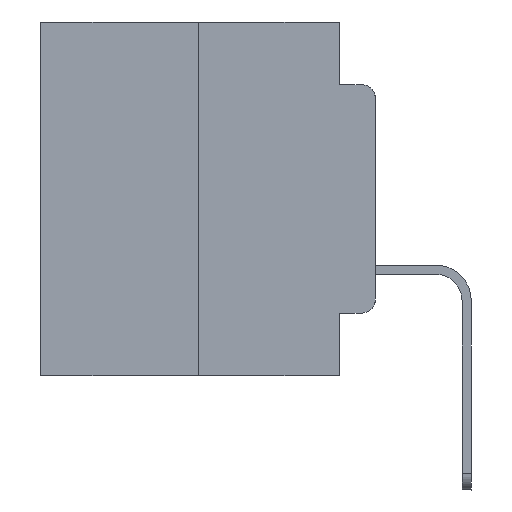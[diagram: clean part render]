
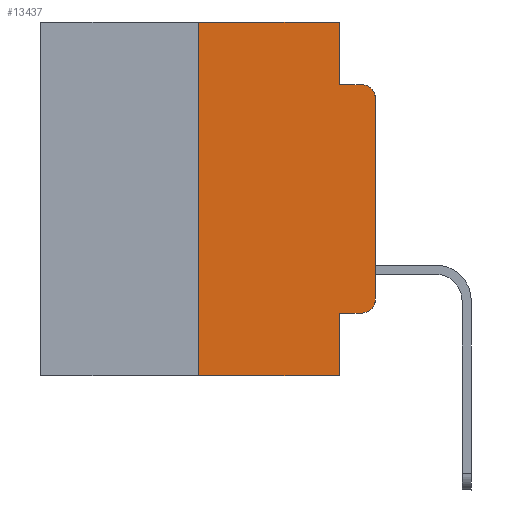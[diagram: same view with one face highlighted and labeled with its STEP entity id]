
A CAD part, left-side view. The second image highlights one B-rep face of the part: STEP entity #13437.
In plain terms, the highlighted planar face has unit normal (-1, 0, 0).
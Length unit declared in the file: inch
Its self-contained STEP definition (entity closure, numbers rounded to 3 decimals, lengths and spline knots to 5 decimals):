
#523 = CARTESIAN_POINT ( 'NONE',  ( 0., 0.02, -0.0885 ) ) ;
#645 = VECTOR ( 'NONE', #2696, 39.37008 ) ;
#682 = VERTEX_POINT ( 'NONE', #3819 ) ;
#1210 = VERTEX_POINT ( 'NONE', #19512 ) ;
#1734 = PLANE ( 'NONE',  #8685 ) ;
#1795 = EDGE_LOOP ( 'NONE', ( #7085, #4631, #19929, #17589, #19676, #7220, #11823, #26872, #26747, #7001 ) ) ;
#2447 = EDGE_CURVE ( 'NONE', #17027, #6965, #3572, .T. ) ;
#2696 = DIRECTION ( 'NONE',  ( 0., -1., 0. ) ) ;
#2859 = VERTEX_POINT ( 'NONE', #14136 ) ;
#2995 = VERTEX_POINT ( 'NONE', #21098 ) ;
#3008 = LINE ( 'NONE', #17358, #15386 ) ;
#3299 = EDGE_CURVE ( 'NONE', #2995, #1210, #4804, .T. ) ;
#3401 = DIRECTION ( 'NONE',  ( 0., -1., 0. ) ) ;
#3572 = LINE ( 'NONE', #23166, #25072 ) ;
#3819 = CARTESIAN_POINT ( 'NONE',  ( 0., 0.25, -0.5 ) ) ;
#4591 = CARTESIAN_POINT ( 'NONE',  ( 0., 0.02, -0.3915 ) ) ;
#4631 = ORIENTED_EDGE ( 'NONE', *, *, #19689, .T. ) ;
#4804 = LINE ( 'NONE', #20510, #16554 ) ;
#5043 = CARTESIAN_POINT ( 'NONE',  ( 0., 0.051, -0.0885 ) ) ;
#6478 = CIRCLE ( 'NONE', #6542, 0.02 ) ;
#6542 = AXIS2_PLACEMENT_3D ( 'NONE', #13864, #15934, #7295 ) ;
#6589 = EDGE_CURVE ( 'NONE', #17250, #19803, #21943, .T. ) ;
#6624 = EDGE_CURVE ( 'NONE', #2859, #8925, #10543, .T. ) ;
#6965 = VERTEX_POINT ( 'NONE', #19039 ) ;
#7001 = ORIENTED_EDGE ( 'NONE', *, *, #10308, .T. ) ;
#7067 = DIRECTION ( 'NONE',  ( 0., 0., -1. ) ) ;
#7085 = ORIENTED_EDGE ( 'NONE', *, *, #3299, .T. ) ;
#7220 = ORIENTED_EDGE ( 'NONE', *, *, #10747, .F. ) ;
#7295 = DIRECTION ( 'NONE',  ( 0., 0., -1. ) ) ;
#8685 = AXIS2_PLACEMENT_3D ( 'NONE', #9784, #13973, #9871 ) ;
#8925 = VERTEX_POINT ( 'NONE', #15623 ) ;
#9784 = CARTESIAN_POINT ( 'NONE',  ( 0., 0.473, 0. ) ) ;
#9871 = DIRECTION ( 'NONE',  ( 0., 0., -1. ) ) ;
#10241 = DIRECTION ( 'NONE',  ( 0., 0., 1. ) ) ;
#10308 = EDGE_CURVE ( 'NONE', #23856, #2995, #23254, .T. ) ;
#10543 = LINE ( 'NONE', #24446, #20632 ) ;
#10747 = EDGE_CURVE ( 'NONE', #682, #17027, #17678, .T. ) ;
#11102 = CARTESIAN_POINT ( 'NONE',  ( 0., 0.051, -0.4115 ) ) ;
#11119 = DIRECTION ( 'NONE',  ( 0., -1., 0. ) ) ;
#11823 = ORIENTED_EDGE ( 'NONE', *, *, #25903, .T. ) ;
#12394 = LINE ( 'NONE', #11102, #645 ) ;
#12458 = EDGE_CURVE ( 'NONE', #2859, #23856, #12394, .T. ) ;
#13437 = ADVANCED_FACE ( 'NONE', ( #26699 ), #1734, .F. ) ;
#13864 = CARTESIAN_POINT ( 'NONE',  ( 0., 0.02, -0.1085 ) ) ;
#13973 = DIRECTION ( 'NONE',  ( 1., 0., 0. ) ) ;
#14027 = DIRECTION ( 'NONE',  ( 0., 0., 1. ) ) ;
#14078 = DIRECTION ( 'NONE',  ( 0., 0., -1. ) ) ;
#14136 = CARTESIAN_POINT ( 'NONE',  ( 0., 0.051, -0.4115 ) ) ;
#14572 = LINE ( 'NONE', #15893, #24664 ) ;
#14951 = DIRECTION ( 'NONE',  ( 0., -1., 0. ) ) ;
#15386 = VECTOR ( 'NONE', #11119, 39.37008 ) ;
#15623 = CARTESIAN_POINT ( 'NONE',  ( 0., 0.051, -0.5 ) ) ;
#15893 = CARTESIAN_POINT ( 'NONE',  ( 0., 0.051, 0. ) ) ;
#15934 = DIRECTION ( 'NONE',  ( -1., 0., 0. ) ) ;
#16407 = VECTOR ( 'NONE', #3401, 39.37008 ) ;
#16450 = AXIS2_PLACEMENT_3D ( 'NONE', #4591, #19170, #7067 ) ;
#16554 = VECTOR ( 'NONE', #10241, 39.37008 ) ;
#16778 = CARTESIAN_POINT ( 'NONE',  ( 0., 0.25, 0. ) ) ;
#17027 = VERTEX_POINT ( 'NONE', #16778 ) ;
#17250 = VERTEX_POINT ( 'NONE', #22443 ) ;
#17358 = CARTESIAN_POINT ( 'NONE',  ( 0., 0.473, -0.5 ) ) ;
#17589 = ORIENTED_EDGE ( 'NONE', *, *, #20681, .F. ) ;
#17678 = LINE ( 'NONE', #25525, #22578 ) ;
#18057 = DIRECTION ( 'NONE',  ( 0., 0., -1. ) ) ;
#19039 = CARTESIAN_POINT ( 'NONE',  ( 0., 0.051, 0. ) ) ;
#19170 = DIRECTION ( 'NONE',  ( -1., 0., 0. ) ) ;
#19512 = CARTESIAN_POINT ( 'NONE',  ( 0., 0., -0.1085 ) ) ;
#19676 = ORIENTED_EDGE ( 'NONE', *, *, #2447, .F. ) ;
#19689 = EDGE_CURVE ( 'NONE', #1210, #19803, #6478, .T. ) ;
#19803 = VERTEX_POINT ( 'NONE', #523 ) ;
#19929 = ORIENTED_EDGE ( 'NONE', *, *, #6589, .F. ) ;
#20510 = CARTESIAN_POINT ( 'NONE',  ( 0., 0., 0. ) ) ;
#20632 = VECTOR ( 'NONE', #14078, 39.37008 ) ;
#20681 = EDGE_CURVE ( 'NONE', #6965, #17250, #14572, .T. ) ;
#20718 = CARTESIAN_POINT ( 'NONE',  ( 0., 0.02, -0.4115 ) ) ;
#21098 = CARTESIAN_POINT ( 'NONE',  ( 0., 0., -0.3915 ) ) ;
#21943 = LINE ( 'NONE', #5043, #16407 ) ;
#22443 = CARTESIAN_POINT ( 'NONE',  ( 0., 0.051, -0.0885 ) ) ;
#22578 = VECTOR ( 'NONE', #14027, 39.37008 ) ;
#23166 = CARTESIAN_POINT ( 'NONE',  ( 0., 0.473, 0. ) ) ;
#23254 = CIRCLE ( 'NONE', #16450, 0.02 ) ;
#23856 = VERTEX_POINT ( 'NONE', #20718 ) ;
#24446 = CARTESIAN_POINT ( 'NONE',  ( 0., 0.051, 0. ) ) ;
#24664 = VECTOR ( 'NONE', #18057, 39.37008 ) ;
#25072 = VECTOR ( 'NONE', #14951, 39.37008 ) ;
#25525 = CARTESIAN_POINT ( 'NONE',  ( 0., 0.25, 0. ) ) ;
#25903 = EDGE_CURVE ( 'NONE', #682, #8925, #3008, .T. ) ;
#26699 = FACE_OUTER_BOUND ( 'NONE', #1795, .T. ) ;
#26747 = ORIENTED_EDGE ( 'NONE', *, *, #12458, .T. ) ;
#26872 = ORIENTED_EDGE ( 'NONE', *, *, #6624, .F. ) ;
